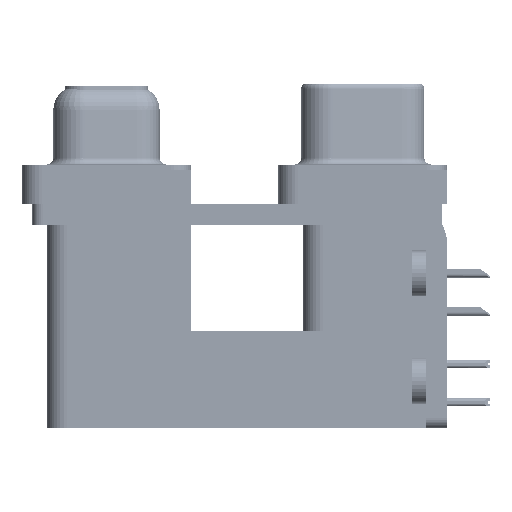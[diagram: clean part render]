
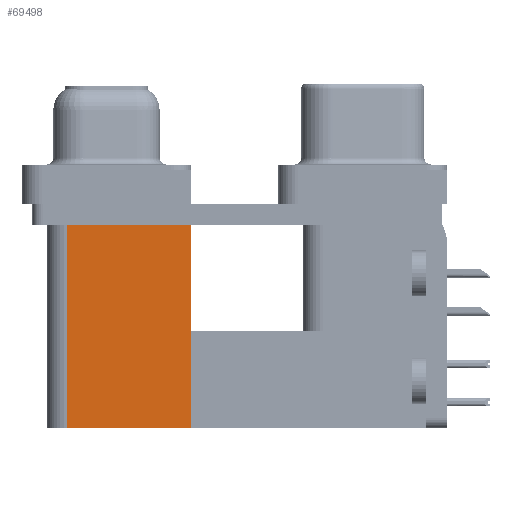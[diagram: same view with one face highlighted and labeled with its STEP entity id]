
A CAD part, left-side view. The second image highlights one B-rep face of the part: STEP entity #69498.
In plain terms, the highlighted planar face has unit normal (-1, 0, 0).
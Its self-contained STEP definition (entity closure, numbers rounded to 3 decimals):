
#2243 = EDGE_CURVE ( 'NONE', #53588, #46215, #7631, .T. ) ;
#3327 = VECTOR ( 'NONE', #46699, 1000. ) ;
#3634 = EDGE_LOOP ( 'NONE', ( #37166, #16141, #12566, #32471 ) ) ;
#3844 = CARTESIAN_POINT ( 'NONE',  ( 3.79, 21.975, -19.2 ) ) ;
#4920 = LINE ( 'NONE', #5264, #61842 ) ;
#5264 = CARTESIAN_POINT ( 'NONE',  ( 3.79, 21.975, -19.2 ) ) ;
#7631 = LINE ( 'NONE', #62288, #3327 ) ;
#8943 = LINE ( 'NONE', #46930, #66904 ) ;
#10021 = CARTESIAN_POINT ( 'NONE',  ( 3.79, 12.775, -2.5 ) ) ;
#10377 = LINE ( 'NONE', #10021, #21698 ) ;
#11677 = CARTESIAN_POINT ( 'NONE',  ( 3.79, 12.775, -19.2 ) ) ;
#12566 = ORIENTED_EDGE ( 'NONE', *, *, #32235, .F. ) ;
#16141 = ORIENTED_EDGE ( 'NONE', *, *, #70195, .F. ) ;
#17489 = AXIS2_PLACEMENT_3D ( 'NONE', #45878, #24213, #46227 ) ;
#19915 = DIRECTION ( 'NONE',  ( 0., 1., 0. ) ) ;
#21698 = VECTOR ( 'NONE', #62912, 1000. ) ;
#24213 = DIRECTION ( 'NONE',  ( 1., 0., 0. ) ) ;
#25370 = VERTEX_POINT ( 'NONE', #3844 ) ;
#26570 = DIRECTION ( 'NONE',  ( 0., 0., 1. ) ) ;
#32235 = EDGE_CURVE ( 'NONE', #53588, #25370, #8943, .T. ) ;
#32465 = CARTESIAN_POINT ( 'NONE',  ( 3.79, 21.975, -2.5 ) ) ;
#32471 = ORIENTED_EDGE ( 'NONE', *, *, #2243, .T. ) ;
#37166 = ORIENTED_EDGE ( 'NONE', *, *, #64235, .T. ) ;
#45878 = CARTESIAN_POINT ( 'NONE',  ( 3.79, 12.775, -19.2 ) ) ;
#46215 = VERTEX_POINT ( 'NONE', #47052 ) ;
#46227 = DIRECTION ( 'NONE',  ( 0., 1., 0. ) ) ;
#46406 = VERTEX_POINT ( 'NONE', #32465 ) ;
#46699 = DIRECTION ( 'NONE',  ( 0., 0., 1. ) ) ;
#46930 = CARTESIAN_POINT ( 'NONE',  ( 3.79, 12.775, -19.2 ) ) ;
#47052 = CARTESIAN_POINT ( 'NONE',  ( 3.79, 12.775, -2.5 ) ) ;
#50169 = PLANE ( 'NONE',  #17489 ) ;
#51538 = FACE_OUTER_BOUND ( 'NONE', #3634, .T. ) ;
#53588 = VERTEX_POINT ( 'NONE', #11677 ) ;
#61842 = VECTOR ( 'NONE', #26570, 1000. ) ;
#62288 = CARTESIAN_POINT ( 'NONE',  ( 3.79, 12.775, -19.2 ) ) ;
#62912 = DIRECTION ( 'NONE',  ( 0., 1., 0. ) ) ;
#64235 = EDGE_CURVE ( 'NONE', #46215, #46406, #10377, .T. ) ;
#66904 = VECTOR ( 'NONE', #19915, 1000. ) ;
#69498 = ADVANCED_FACE ( 'NONE', ( #51538 ), #50169, .F. ) ;
#70195 = EDGE_CURVE ( 'NONE', #25370, #46406, #4920, .T. ) ;
